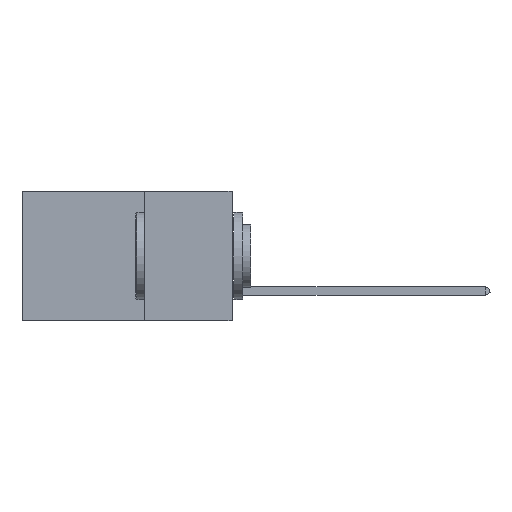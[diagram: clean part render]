
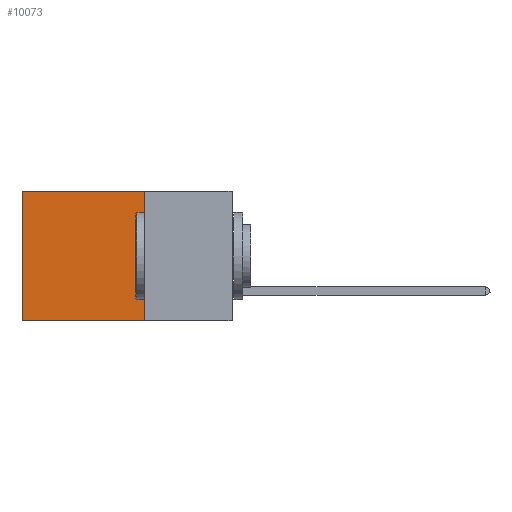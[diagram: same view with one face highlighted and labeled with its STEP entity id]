
A CAD part, left-side view. The second image highlights one B-rep face of the part: STEP entity #10073.
In plain terms, the highlighted planar face has unit normal (-1, 0, 0).
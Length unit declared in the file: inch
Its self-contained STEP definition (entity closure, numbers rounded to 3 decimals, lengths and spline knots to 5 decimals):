
#1468 = LINE ( 'NONE', #15996, #7400 ) ;
#2454 = DIRECTION ( 'NONE',  ( 0., 0., -1. ) ) ;
#2523 = VECTOR ( 'NONE', #25519, 39.37008 ) ;
#3912 = CARTESIAN_POINT ( 'NONE',  ( 0.2875, 0.25, -0.37 ) ) ;
#4188 = LINE ( 'NONE', #4335, #2523 ) ;
#4335 = CARTESIAN_POINT ( 'NONE',  ( 0.2875, 0.25, 0. ) ) ;
#5958 = LINE ( 'NONE', #8234, #16160 ) ;
#7400 = VECTOR ( 'NONE', #20080, 39.37008 ) ;
#7579 = CARTESIAN_POINT ( 'NONE',  ( 0.2875, 0.25, 0. ) ) ;
#7781 = ORIENTED_EDGE ( 'NONE', *, *, #10044, .T. ) ;
#8051 = EDGE_CURVE ( 'NONE', #18134, #19333, #5958, .T. ) ;
#8234 = CARTESIAN_POINT ( 'NONE',  ( 0.2875, 0.25, -0.37 ) ) ;
#8543 = CARTESIAN_POINT ( 'NONE',  ( 0.2875, 0.6, -0.37 ) ) ;
#8719 = CARTESIAN_POINT ( 'NONE',  ( 0.2875, 0.25, 0. ) ) ;
#8738 = EDGE_LOOP ( 'NONE', ( #21260, #23541, #18353, #7781 ) ) ;
#9050 = VERTEX_POINT ( 'NONE', #7579 ) ;
#9494 = VERTEX_POINT ( 'NONE', #16565 ) ;
#10044 = EDGE_CURVE ( 'NONE', #9050, #9494, #4188, .T. ) ;
#10073 = ADVANCED_FACE ( 'NONE', ( #24311 ), #19416, .F. ) ;
#11089 = CARTESIAN_POINT ( 'NONE',  ( 0.2875, 0.6, 0. ) ) ;
#15996 = CARTESIAN_POINT ( 'NONE',  ( 0.2875, 0.25, 0. ) ) ;
#16160 = VECTOR ( 'NONE', #20306, 39.37008 ) ;
#16565 = CARTESIAN_POINT ( 'NONE',  ( 0.2875, 0.6, 0. ) ) ;
#18134 = VERTEX_POINT ( 'NONE', #3912 ) ;
#18353 = ORIENTED_EDGE ( 'NONE', *, *, #22250, .F. ) ;
#18969 = DIRECTION ( 'NONE',  ( 0., 0., -1. ) ) ;
#19145 = DIRECTION ( 'NONE',  ( 1., 0., 0. ) ) ;
#19333 = VERTEX_POINT ( 'NONE', #8543 ) ;
#19416 = PLANE ( 'NONE',  #25749 ) ;
#19450 = LINE ( 'NONE', #11089, #21738 ) ;
#19548 = EDGE_CURVE ( 'NONE', #9494, #19333, #19450, .T. ) ;
#20080 = DIRECTION ( 'NONE',  ( 0., 0., -1. ) ) ;
#20306 = DIRECTION ( 'NONE',  ( 0., 1., 0. ) ) ;
#21260 = ORIENTED_EDGE ( 'NONE', *, *, #19548, .T. ) ;
#21738 = VECTOR ( 'NONE', #18969, 39.37008 ) ;
#22250 = EDGE_CURVE ( 'NONE', #9050, #18134, #1468, .T. ) ;
#23541 = ORIENTED_EDGE ( 'NONE', *, *, #8051, .F. ) ;
#24311 = FACE_OUTER_BOUND ( 'NONE', #8738, .T. ) ;
#25519 = DIRECTION ( 'NONE',  ( 0., 1., 0. ) ) ;
#25749 = AXIS2_PLACEMENT_3D ( 'NONE', #8719, #19145, #2454 ) ;
